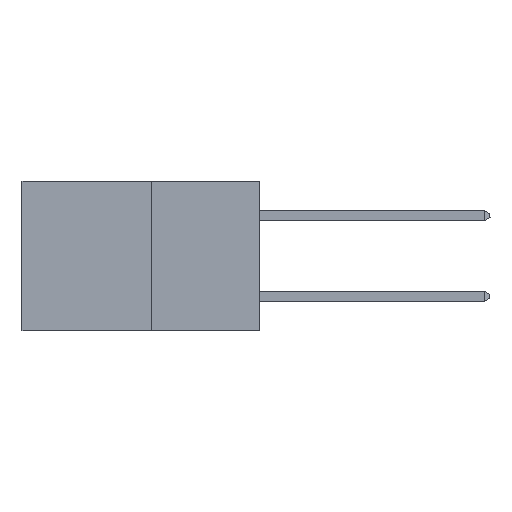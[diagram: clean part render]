
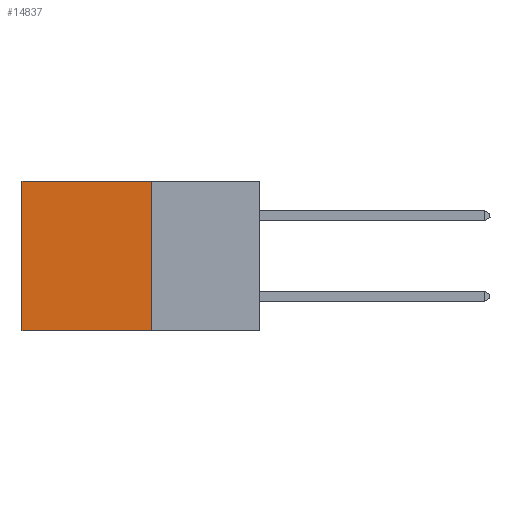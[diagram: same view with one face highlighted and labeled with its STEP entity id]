
A CAD part, left-side view. The second image highlights one B-rep face of the part: STEP entity #14837.
In plain terms, the highlighted planar face has unit normal (-1, 0, 0).
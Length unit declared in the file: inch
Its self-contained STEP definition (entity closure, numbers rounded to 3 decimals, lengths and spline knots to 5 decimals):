
#67 = ORIENTED_EDGE ( 'NONE', *, *, #10156, .T. ) ;
#1143 = VERTEX_POINT ( 'NONE', #2712 ) ;
#2510 = CARTESIAN_POINT ( 'NONE',  ( 0.277, 0.27, -0.37 ) ) ;
#2712 = CARTESIAN_POINT ( 'NONE',  ( 0.277, 0.59, 0. ) ) ;
#2716 = ORIENTED_EDGE ( 'NONE', *, *, #5440, .T. ) ;
#3345 = LINE ( 'NONE', #14491, #16098 ) ;
#3698 = ORIENTED_EDGE ( 'NONE', *, *, #5293, .F. ) ;
#3802 = DIRECTION ( 'NONE',  ( 0., 1., 0. ) ) ;
#4093 = VERTEX_POINT ( 'NONE', #16112 ) ;
#4687 = ORIENTED_EDGE ( 'NONE', *, *, #14354, .F. ) ;
#4703 = CARTESIAN_POINT ( 'NONE',  ( 0.277, 0.59, -0.37 ) ) ;
#4991 = VECTOR ( 'NONE', #3802, 39.37008 ) ;
#5293 = EDGE_CURVE ( 'NONE', #13270, #4093, #9151, .T. ) ;
#5440 = EDGE_CURVE ( 'NONE', #1143, #8958, #3345, .T. ) ;
#5803 = VECTOR ( 'NONE', #6529, 39.37008 ) ;
#5839 = CARTESIAN_POINT ( 'NONE',  ( 0.277, 0.27, 0. ) ) ;
#6529 = DIRECTION ( 'NONE',  ( 0., 0., -1. ) ) ;
#7040 = DIRECTION ( 'NONE',  ( 0., 1., 0. ) ) ;
#7206 = CARTESIAN_POINT ( 'NONE',  ( 0.277, 0.27, -0.37 ) ) ;
#7250 = DIRECTION ( 'NONE',  ( 0., 0., -1. ) ) ;
#8313 = CARTESIAN_POINT ( 'NONE',  ( 0.277, 0.27, 0. ) ) ;
#8324 = VECTOR ( 'NONE', #7040, 39.37008 ) ;
#8385 = LINE ( 'NONE', #2510, #4991 ) ;
#8761 = FACE_OUTER_BOUND ( 'NONE', #11791, .T. ) ;
#8958 = VERTEX_POINT ( 'NONE', #4703 ) ;
#9151 = LINE ( 'NONE', #7206, #5803 ) ;
#9687 = CARTESIAN_POINT ( 'NONE',  ( 0.277, 0.27, -0.37 ) ) ;
#10156 = EDGE_CURVE ( 'NONE', #13270, #1143, #11201, .T. ) ;
#11201 = LINE ( 'NONE', #8313, #8324 ) ;
#11791 = EDGE_LOOP ( 'NONE', ( #2716, #4687, #3698, #67 ) ) ;
#12464 = AXIS2_PLACEMENT_3D ( 'NONE', #9687, #14559, #7250 ) ;
#13270 = VERTEX_POINT ( 'NONE', #5839 ) ;
#13362 = PLANE ( 'NONE',  #12464 ) ;
#14179 = DIRECTION ( 'NONE',  ( 0., 0., -1. ) ) ;
#14354 = EDGE_CURVE ( 'NONE', #4093, #8958, #8385, .T. ) ;
#14491 = CARTESIAN_POINT ( 'NONE',  ( 0.277, 0.59, -0.37 ) ) ;
#14559 = DIRECTION ( 'NONE',  ( 1., 0., 0. ) ) ;
#14837 = ADVANCED_FACE ( 'NONE', ( #8761 ), #13362, .F. ) ;
#16098 = VECTOR ( 'NONE', #14179, 39.37008 ) ;
#16112 = CARTESIAN_POINT ( 'NONE',  ( 0.277, 0.27, -0.37 ) ) ;
